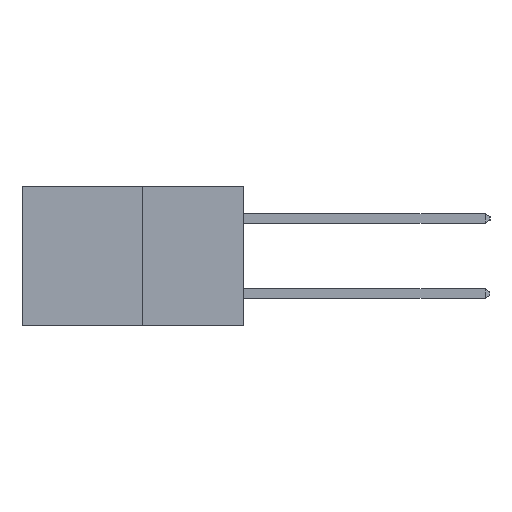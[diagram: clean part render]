
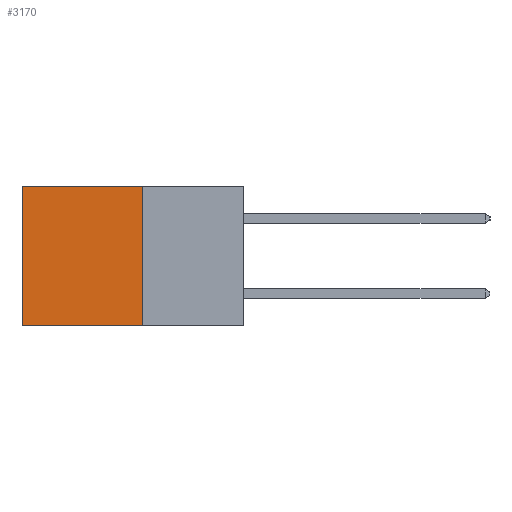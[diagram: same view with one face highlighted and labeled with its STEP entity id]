
A CAD part, left-side view. The second image highlights one B-rep face of the part: STEP entity #3170.
In plain terms, the highlighted planar face has unit normal (-1, 0, 0).
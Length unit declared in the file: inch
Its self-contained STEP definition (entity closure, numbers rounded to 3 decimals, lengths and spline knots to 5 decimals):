
#201 = CARTESIAN_POINT ( 'NONE',  ( 0.277, 0.27, -0.37 ) ) ;
#350 = DIRECTION ( 'NONE',  ( 0., 0., -1. ) ) ;
#425 = CARTESIAN_POINT ( 'NONE',  ( 0.277, 0.27, -0.37 ) ) ;
#931 = EDGE_CURVE ( 'NONE', #4814, #5277, #5355, .T. ) ;
#1080 = ORIENTED_EDGE ( 'NONE', *, *, #931, .T. ) ;
#1560 = LINE ( 'NONE', #5571, #4977 ) ;
#1647 = AXIS2_PLACEMENT_3D ( 'NONE', #4738, #2241, #8237 ) ;
#1873 = VERTEX_POINT ( 'NONE', #7480 ) ;
#1945 = DIRECTION ( 'NONE',  ( 0., 0., -1. ) ) ;
#2241 = DIRECTION ( 'NONE',  ( 1., 0., 0. ) ) ;
#2562 = CARTESIAN_POINT ( 'NONE',  ( 0.277, 0.59, -0.37 ) ) ;
#3170 = ADVANCED_FACE ( 'NONE', ( #7880 ), #4818, .F. ) ;
#3188 = CARTESIAN_POINT ( 'NONE',  ( 0.277, 0.59, -0.37 ) ) ;
#3331 = EDGE_CURVE ( 'NONE', #1873, #5277, #6393, .T. ) ;
#3709 = EDGE_CURVE ( 'NONE', #6500, #1873, #7422, .T. ) ;
#3881 = DIRECTION ( 'NONE',  ( 0., 1., 0. ) ) ;
#4738 = CARTESIAN_POINT ( 'NONE',  ( 0.277, 0.27, -0.37 ) ) ;
#4814 = VERTEX_POINT ( 'NONE', #7848 ) ;
#4818 = PLANE ( 'NONE',  #1647 ) ;
#4977 = VECTOR ( 'NONE', #5449, 39.37008 ) ;
#5099 = EDGE_CURVE ( 'NONE', #6500, #4814, #1560, .T. ) ;
#5277 = VERTEX_POINT ( 'NONE', #3188 ) ;
#5355 = LINE ( 'NONE', #2562, #6847 ) ;
#5449 = DIRECTION ( 'NONE',  ( 0., 1., 0. ) ) ;
#5470 = ORIENTED_EDGE ( 'NONE', *, *, #3709, .F. ) ;
#5503 = ORIENTED_EDGE ( 'NONE', *, *, #3331, .F. ) ;
#5571 = CARTESIAN_POINT ( 'NONE',  ( 0.277, 0.27, 0. ) ) ;
#5873 = VECTOR ( 'NONE', #1945, 39.37008 ) ;
#6393 = LINE ( 'NONE', #201, #7695 ) ;
#6486 = ORIENTED_EDGE ( 'NONE', *, *, #5099, .T. ) ;
#6500 = VERTEX_POINT ( 'NONE', #8622 ) ;
#6847 = VECTOR ( 'NONE', #350, 39.37008 ) ;
#7422 = LINE ( 'NONE', #425, #5873 ) ;
#7480 = CARTESIAN_POINT ( 'NONE',  ( 0.277, 0.27, -0.37 ) ) ;
#7695 = VECTOR ( 'NONE', #3881, 39.37008 ) ;
#7848 = CARTESIAN_POINT ( 'NONE',  ( 0.277, 0.59, 0. ) ) ;
#7880 = FACE_OUTER_BOUND ( 'NONE', #7935, .T. ) ;
#7935 = EDGE_LOOP ( 'NONE', ( #1080, #5503, #5470, #6486 ) ) ;
#8237 = DIRECTION ( 'NONE',  ( 0., 0., -1. ) ) ;
#8622 = CARTESIAN_POINT ( 'NONE',  ( 0.277, 0.27, 0. ) ) ;
